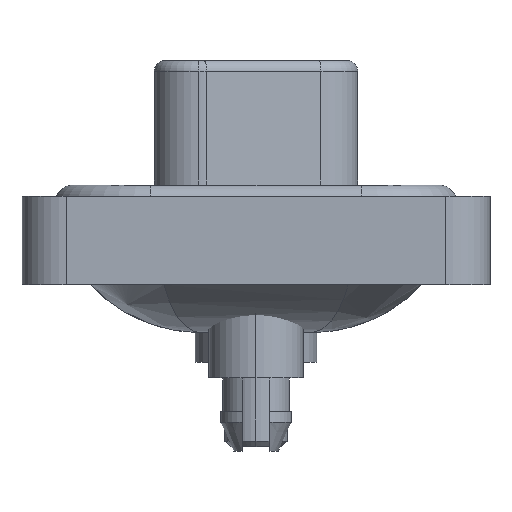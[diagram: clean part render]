
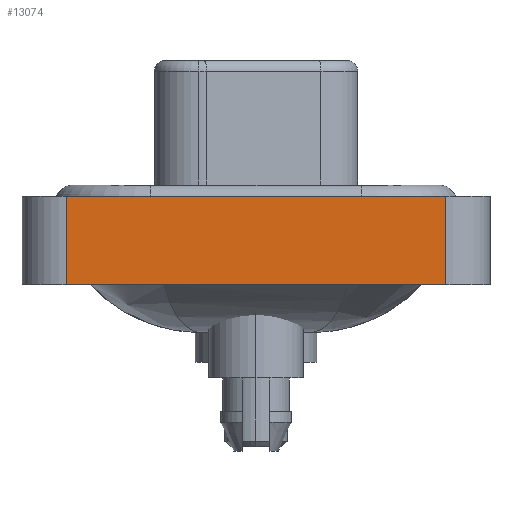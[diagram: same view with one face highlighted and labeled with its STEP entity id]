
A CAD part, left-side view. The second image highlights one B-rep face of the part: STEP entity #13074.
In plain terms, the highlighted planar face has unit normal (-1, 0, 0).
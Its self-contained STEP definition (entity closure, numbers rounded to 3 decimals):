
#543 = DIRECTION ( 'NONE',  ( 0., -1., 0. ) ) ;
#1489 = CARTESIAN_POINT ( 'NONE',  ( -7.3, -8.55, -3.6 ) ) ;
#2364 = CARTESIAN_POINT ( 'NONE',  ( -7.3, -8.55, -3.6 ) ) ;
#3175 = VERTEX_POINT ( 'NONE', #21508 ) ;
#3320 = VERTEX_POINT ( 'NONE', #16125 ) ;
#3324 = DIRECTION ( 'NONE',  ( -1., 0., 0. ) ) ;
#4441 = LINE ( 'NONE', #20953, #23124 ) ;
#5187 = EDGE_CURVE ( 'NONE', #3320, #12784, #4441, .T. ) ;
#6420 = LINE ( 'NONE', #2364, #10405 ) ;
#6480 = VECTOR ( 'NONE', #24063, 1000. ) ;
#6956 = ORIENTED_EDGE ( 'NONE', *, *, #14779, .F. ) ;
#7119 = DIRECTION ( 'NONE',  ( 0., 0., 1. ) ) ;
#7362 = EDGE_CURVE ( 'NONE', #21912, #12784, #17115, .T. ) ;
#10309 = ORIENTED_EDGE ( 'NONE', *, *, #5187, .T. ) ;
#10405 = VECTOR ( 'NONE', #543, 1000. ) ;
#11131 = DIRECTION ( 'NONE',  ( 0., -1., 0. ) ) ;
#11249 = CARTESIAN_POINT ( 'NONE',  ( -7.3, -8.55, 0.4 ) ) ;
#12552 = CARTESIAN_POINT ( 'NONE',  ( -7.3, -8.55, 0.4 ) ) ;
#12784 = VERTEX_POINT ( 'NONE', #12552 ) ;
#13074 = ADVANCED_FACE ( 'NONE', ( #19953 ), #18244, .T. ) ;
#13863 = ORIENTED_EDGE ( 'NONE', *, *, #7362, .F. ) ;
#14779 = EDGE_CURVE ( 'NONE', #3175, #21912, #19904, .T. ) ;
#14890 = CARTESIAN_POINT ( 'NONE',  ( -7.3, 8.55, -3.6 ) ) ;
#15352 = EDGE_CURVE ( 'NONE', #3175, #3320, #6420, .T. ) ;
#16125 = CARTESIAN_POINT ( 'NONE',  ( -7.3, -8.55, -3.6 ) ) ;
#17069 = EDGE_LOOP ( 'NONE', ( #10309, #13863, #6956, #21383 ) ) ;
#17115 = LINE ( 'NONE', #11249, #22702 ) ;
#18244 = PLANE ( 'NONE',  #22828 ) ;
#19749 = CARTESIAN_POINT ( 'NONE',  ( -7.3, 8.55, 0.4 ) ) ;
#19904 = LINE ( 'NONE', #14890, #6480 ) ;
#19953 = FACE_OUTER_BOUND ( 'NONE', #17069, .T. ) ;
#20953 = CARTESIAN_POINT ( 'NONE',  ( -7.3, -8.55, -3.6 ) ) ;
#21383 = ORIENTED_EDGE ( 'NONE', *, *, #15352, .T. ) ;
#21435 = DIRECTION ( 'NONE',  ( 0., 0., 1. ) ) ;
#21508 = CARTESIAN_POINT ( 'NONE',  ( -7.3, 8.55, -3.6 ) ) ;
#21912 = VERTEX_POINT ( 'NONE', #19749 ) ;
#22702 = VECTOR ( 'NONE', #11131, 1000. ) ;
#22828 = AXIS2_PLACEMENT_3D ( 'NONE', #1489, #3324, #7119 ) ;
#23124 = VECTOR ( 'NONE', #21435, 1000. ) ;
#24063 = DIRECTION ( 'NONE',  ( 0., 0., 1. ) ) ;
